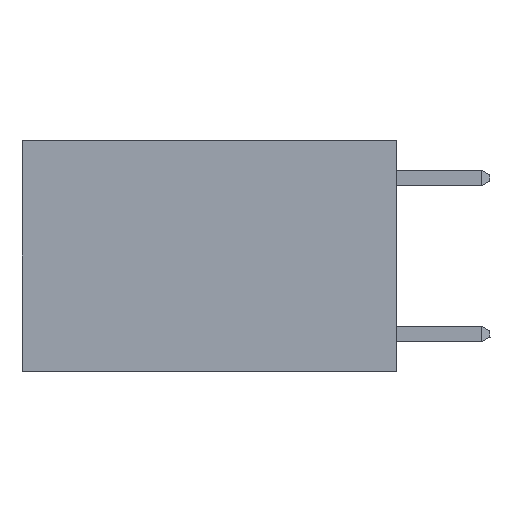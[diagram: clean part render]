
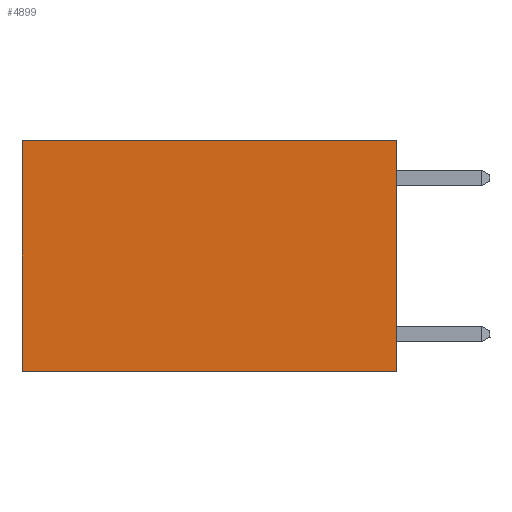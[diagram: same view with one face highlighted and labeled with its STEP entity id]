
A CAD part, left-side view. The second image highlights one B-rep face of the part: STEP entity #4899.
In plain terms, the highlighted planar face has unit normal (-1, 0, 0).
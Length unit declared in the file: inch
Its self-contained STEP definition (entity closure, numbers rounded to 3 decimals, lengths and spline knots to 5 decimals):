
#454 = DIRECTION ( 'NONE',  ( 0., 0., -1. ) ) ;
#492 = AXIS2_PLACEMENT_3D ( 'NONE', #5248, #5938, #1719 ) ;
#509 = CARTESIAN_POINT ( 'NONE',  ( 0.2625, 0., 0. ) ) ;
#1719 = DIRECTION ( 'NONE',  ( 0., 0., -1. ) ) ;
#2199 = VECTOR ( 'NONE', #5443, 39.37008 ) ;
#2424 = LINE ( 'NONE', #8156, #2199 ) ;
#3087 = CARTESIAN_POINT ( 'NONE',  ( 0.2625, 0.6, 0. ) ) ;
#3300 = VECTOR ( 'NONE', #6274, 39.37008 ) ;
#3384 = CARTESIAN_POINT ( 'NONE',  ( 0.2625, 0., -0.37 ) ) ;
#3744 = EDGE_CURVE ( 'NONE', #6493, #8968, #9022, .T. ) ;
#3869 = EDGE_CURVE ( 'NONE', #8968, #8357, #8451, .T. ) ;
#4365 = ORIENTED_EDGE ( 'NONE', *, *, #9019, .T. ) ;
#4384 = VERTEX_POINT ( 'NONE', #3087 ) ;
#4560 = PLANE ( 'NONE',  #492 ) ;
#4801 = ORIENTED_EDGE ( 'NONE', *, *, #7632, .T. ) ;
#4807 = CARTESIAN_POINT ( 'NONE',  ( 0.2625, 0.6, -0.37 ) ) ;
#4899 = ADVANCED_FACE ( 'NONE', ( #5137 ), #4560, .F. ) ;
#5137 = FACE_OUTER_BOUND ( 'NONE', #7021, .T. ) ;
#5248 = CARTESIAN_POINT ( 'NONE',  ( 0.2625, 0., 0. ) ) ;
#5383 = LINE ( 'NONE', #5538, #3300 ) ;
#5443 = DIRECTION ( 'NONE',  ( 0., 1., 0. ) ) ;
#5480 = VECTOR ( 'NONE', #454, 39.37008 ) ;
#5538 = CARTESIAN_POINT ( 'NONE',  ( 0.2625, 0.6, 0. ) ) ;
#5938 = DIRECTION ( 'NONE',  ( 1., 0., 0. ) ) ;
#6223 = ORIENTED_EDGE ( 'NONE', *, *, #3869, .F. ) ;
#6274 = DIRECTION ( 'NONE',  ( 0., 0., -1. ) ) ;
#6334 = CARTESIAN_POINT ( 'NONE',  ( 0.2625, 0., 0. ) ) ;
#6493 = VERTEX_POINT ( 'NONE', #6334 ) ;
#7021 = EDGE_LOOP ( 'NONE', ( #4365, #6223, #8205, #4801 ) ) ;
#7632 = EDGE_CURVE ( 'NONE', #6493, #4384, #2424, .T. ) ;
#8156 = CARTESIAN_POINT ( 'NONE',  ( 0.2625, 0., 0. ) ) ;
#8205 = ORIENTED_EDGE ( 'NONE', *, *, #3744, .F. ) ;
#8243 = VECTOR ( 'NONE', #8568, 39.37008 ) ;
#8357 = VERTEX_POINT ( 'NONE', #4807 ) ;
#8451 = LINE ( 'NONE', #8556, #8243 ) ;
#8556 = CARTESIAN_POINT ( 'NONE',  ( 0.2625, 0., -0.37 ) ) ;
#8568 = DIRECTION ( 'NONE',  ( 0., 1., 0. ) ) ;
#8968 = VERTEX_POINT ( 'NONE', #3384 ) ;
#9019 = EDGE_CURVE ( 'NONE', #4384, #8357, #5383, .T. ) ;
#9022 = LINE ( 'NONE', #509, #5480 ) ;
